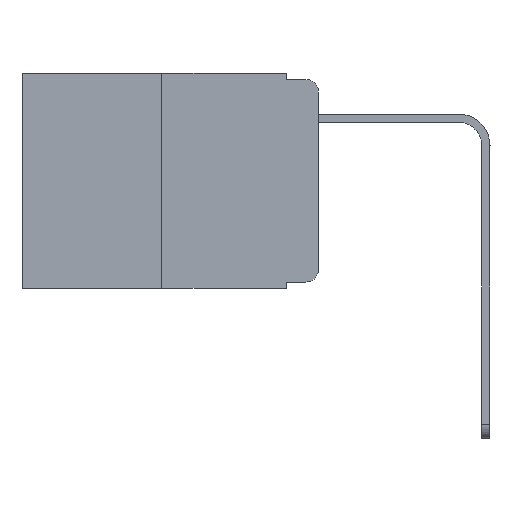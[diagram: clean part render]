
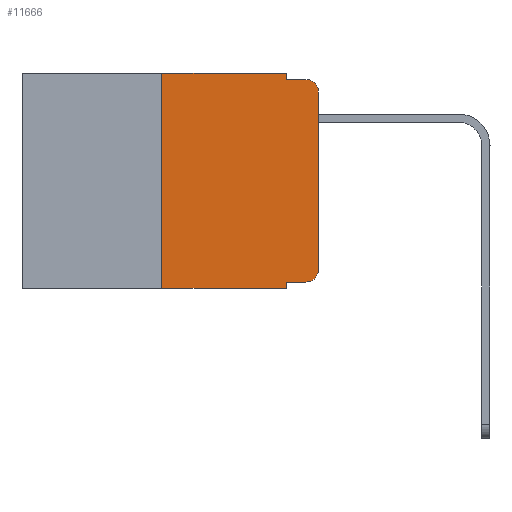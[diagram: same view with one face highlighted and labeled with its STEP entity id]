
A CAD part, left-side view. The second image highlights one B-rep face of the part: STEP entity #11666.
In plain terms, the highlighted planar face has unit normal (-1, 0, 0).
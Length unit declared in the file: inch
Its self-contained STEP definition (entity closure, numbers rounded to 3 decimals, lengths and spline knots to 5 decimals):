
#243 = DIRECTION ( 'NONE',  ( 0., -1., 0. ) ) ;
#946 = EDGE_CURVE ( 'NONE', #11378, #6816, #10850, .T. ) ;
#1013 = AXIS2_PLACEMENT_3D ( 'NONE', #9657, #3800, #5994 ) ;
#1364 = VECTOR ( 'NONE', #2680, 39.37008 ) ;
#1641 = ORIENTED_EDGE ( 'NONE', *, *, #4578, .T. ) ;
#1805 = CARTESIAN_POINT ( 'NONE',  ( 0., 0., -0.313 ) ) ;
#2021 = EDGE_CURVE ( 'NONE', #2039, #5686, #13293, .T. ) ;
#2033 = EDGE_CURVE ( 'NONE', #8405, #15367, #8211, .T. ) ;
#2039 = VERTEX_POINT ( 'NONE', #15501 ) ;
#2100 = CARTESIAN_POINT ( 'NONE',  ( 0., 0.051, -0.333 ) ) ;
#2139 = DIRECTION ( 'NONE',  ( 0., 0., -1. ) ) ;
#2220 = LINE ( 'NONE', #14408, #15553 ) ;
#2244 = VERTEX_POINT ( 'NONE', #13352 ) ;
#2512 = DIRECTION ( 'NONE',  ( 1., 0., 0. ) ) ;
#2680 = DIRECTION ( 'NONE',  ( 0., 0., -1. ) ) ;
#3137 = LINE ( 'NONE', #10174, #7152 ) ;
#3800 = DIRECTION ( 'NONE',  ( -1., 0., 0. ) ) ;
#4190 = ORIENTED_EDGE ( 'NONE', *, *, #9659, .T. ) ;
#4578 = EDGE_CURVE ( 'NONE', #8405, #6087, #10334, .T. ) ;
#4660 = CARTESIAN_POINT ( 'NONE',  ( 0., 0.02, -0.03 ) ) ;
#4887 = CARTESIAN_POINT ( 'NONE',  ( 0., 0.473, 0. ) ) ;
#5283 = LINE ( 'NONE', #9581, #14168 ) ;
#5344 = AXIS2_PLACEMENT_3D ( 'NONE', #4887, #2512, #11362 ) ;
#5561 = VERTEX_POINT ( 'NONE', #14787 ) ;
#5606 = CARTESIAN_POINT ( 'NONE',  ( 0., 0.02, -0.333 ) ) ;
#5686 = VERTEX_POINT ( 'NONE', #7366 ) ;
#5994 = DIRECTION ( 'NONE',  ( 0., 0., -1. ) ) ;
#6040 = ORIENTED_EDGE ( 'NONE', *, *, #9084, .F. ) ;
#6087 = VERTEX_POINT ( 'NONE', #5606 ) ;
#6392 = ORIENTED_EDGE ( 'NONE', *, *, #9941, .F. ) ;
#6424 = DIRECTION ( 'NONE',  ( 0., -1., 0. ) ) ;
#6439 = DIRECTION ( 'NONE',  ( 0., -1., 0. ) ) ;
#6496 = DIRECTION ( 'NONE',  ( 0., 0., 1. ) ) ;
#6816 = VERTEX_POINT ( 'NONE', #8466 ) ;
#6844 = ORIENTED_EDGE ( 'NONE', *, *, #15245, .T. ) ;
#6882 = AXIS2_PLACEMENT_3D ( 'NONE', #4660, #16220, #9850 ) ;
#7152 = VECTOR ( 'NONE', #6439, 39.37008 ) ;
#7224 = VECTOR ( 'NONE', #12642, 39.37008 ) ;
#7366 = CARTESIAN_POINT ( 'NONE',  ( 0., 0.25, 0. ) ) ;
#7766 = ORIENTED_EDGE ( 'NONE', *, *, #7850, .T. ) ;
#7850 = EDGE_CURVE ( 'NONE', #12735, #11378, #9247, .T. ) ;
#7903 = FACE_OUTER_BOUND ( 'NONE', #15789, .T. ) ;
#8211 = LINE ( 'NONE', #14201, #1364 ) ;
#8226 = DIRECTION ( 'NONE',  ( 0., -1., 0. ) ) ;
#8405 = VERTEX_POINT ( 'NONE', #2100 ) ;
#8466 = CARTESIAN_POINT ( 'NONE',  ( 0., 0.02, -0.01 ) ) ;
#9084 = EDGE_CURVE ( 'NONE', #5561, #2244, #11419, .T. ) ;
#9247 = LINE ( 'NONE', #13973, #7224 ) ;
#9581 = CARTESIAN_POINT ( 'NONE',  ( 0., 0.051, -0.01 ) ) ;
#9657 = CARTESIAN_POINT ( 'NONE',  ( 0., 0.02, -0.313 ) ) ;
#9659 = EDGE_CURVE ( 'NONE', #6087, #12735, #10974, .T. ) ;
#9801 = CARTESIAN_POINT ( 'NONE',  ( 0., 0.051, 0. ) ) ;
#9850 = DIRECTION ( 'NONE',  ( 0., 0., -1. ) ) ;
#9941 = EDGE_CURVE ( 'NONE', #2244, #6816, #5283, .T. ) ;
#10174 = CARTESIAN_POINT ( 'NONE',  ( 0., 0.473, -0.343 ) ) ;
#10334 = LINE ( 'NONE', #14128, #16241 ) ;
#10506 = CARTESIAN_POINT ( 'NONE',  ( 0., 0.051, -0.343 ) ) ;
#10850 = CIRCLE ( 'NONE', #6882, 0.02 ) ;
#10974 = CIRCLE ( 'NONE', #1013, 0.02 ) ;
#11362 = DIRECTION ( 'NONE',  ( 0., 0., -1. ) ) ;
#11378 = VERTEX_POINT ( 'NONE', #14446 ) ;
#11419 = LINE ( 'NONE', #9801, #12674 ) ;
#11666 = ADVANCED_FACE ( 'NONE', ( #7903 ), #16715, .F. ) ;
#12026 = ORIENTED_EDGE ( 'NONE', *, *, #946, .T. ) ;
#12582 = EDGE_CURVE ( 'NONE', #5686, #5561, #2220, .T. ) ;
#12642 = DIRECTION ( 'NONE',  ( 0., 0., 1. ) ) ;
#12674 = VECTOR ( 'NONE', #2139, 39.37008 ) ;
#12683 = VECTOR ( 'NONE', #6496, 39.37008 ) ;
#12735 = VERTEX_POINT ( 'NONE', #1805 ) ;
#12805 = CARTESIAN_POINT ( 'NONE',  ( 0., 0.25, 0. ) ) ;
#12862 = ORIENTED_EDGE ( 'NONE', *, *, #12582, .F. ) ;
#13293 = LINE ( 'NONE', #12805, #12683 ) ;
#13352 = CARTESIAN_POINT ( 'NONE',  ( 0., 0.051, -0.01 ) ) ;
#13973 = CARTESIAN_POINT ( 'NONE',  ( 0., 0., 0. ) ) ;
#14128 = CARTESIAN_POINT ( 'NONE',  ( 0., 0.051, -0.333 ) ) ;
#14168 = VECTOR ( 'NONE', #8226, 39.37008 ) ;
#14201 = CARTESIAN_POINT ( 'NONE',  ( 0., 0.051, 0. ) ) ;
#14205 = ORIENTED_EDGE ( 'NONE', *, *, #2033, .F. ) ;
#14408 = CARTESIAN_POINT ( 'NONE',  ( 0., 0.473, 0. ) ) ;
#14446 = CARTESIAN_POINT ( 'NONE',  ( 0., 0., -0.03 ) ) ;
#14787 = CARTESIAN_POINT ( 'NONE',  ( 0., 0.051, 0. ) ) ;
#15245 = EDGE_CURVE ( 'NONE', #2039, #15367, #3137, .T. ) ;
#15367 = VERTEX_POINT ( 'NONE', #10506 ) ;
#15498 = ORIENTED_EDGE ( 'NONE', *, *, #2021, .F. ) ;
#15501 = CARTESIAN_POINT ( 'NONE',  ( 0., 0.25, -0.343 ) ) ;
#15553 = VECTOR ( 'NONE', #243, 39.37008 ) ;
#15789 = EDGE_LOOP ( 'NONE', ( #7766, #12026, #6392, #6040, #12862, #15498, #6844, #14205, #1641, #4190 ) ) ;
#16220 = DIRECTION ( 'NONE',  ( -1., 0., 0. ) ) ;
#16241 = VECTOR ( 'NONE', #6424, 39.37008 ) ;
#16715 = PLANE ( 'NONE',  #5344 ) ;
